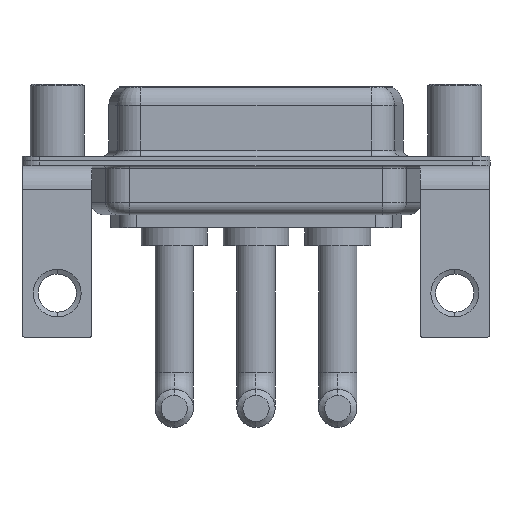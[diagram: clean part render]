
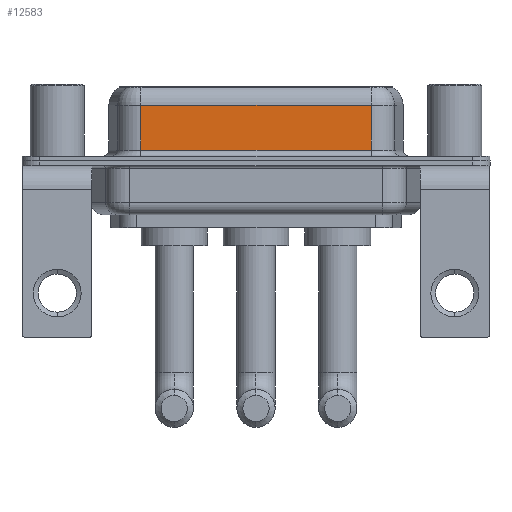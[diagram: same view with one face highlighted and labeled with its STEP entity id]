
A CAD part, front view. The second image highlights one B-rep face of the part: STEP entity #12583.
In plain terms, the highlighted planar face has unit normal (0, -1, 0).
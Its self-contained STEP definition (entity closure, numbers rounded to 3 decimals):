
#270 = VERTEX_POINT ( 'NONE', #8529 ) ;
#632 = EDGE_LOOP ( 'NONE', ( #10201, #5045, #6420, #14072 ) ) ;
#1695 = EDGE_CURVE ( 'NONE', #270, #7792, #4351, .T. ) ;
#2685 = DIRECTION ( 'NONE',  ( 0., 0., 1. ) ) ;
#2960 = CARTESIAN_POINT ( 'NONE',  ( 7.013, -3.95, 4.65 ) ) ;
#3177 = LINE ( 'NONE', #5788, #10766 ) ;
#4142 = CARTESIAN_POINT ( 'NONE',  ( 26.287, -3.95, 0.9 ) ) ;
#4351 = LINE ( 'NONE', #6605, #9673 ) ;
#4959 = AXIS2_PLACEMENT_3D ( 'NONE', #8014, #6900, #2685 ) ;
#5045 = ORIENTED_EDGE ( 'NONE', *, *, #1695, .T. ) ;
#5705 = FACE_OUTER_BOUND ( 'NONE', #632, .T. ) ;
#5788 = CARTESIAN_POINT ( 'NONE',  ( 26.287, -3.95, 6.4 ) ) ;
#6192 = EDGE_CURVE ( 'NONE', #270, #11285, #3177, .T. ) ;
#6420 = ORIENTED_EDGE ( 'NONE', *, *, #8522, .T. ) ;
#6605 = CARTESIAN_POINT ( 'NONE',  ( 26.287, -3.95, 4.65 ) ) ;
#6739 = VERTEX_POINT ( 'NONE', #7516 ) ;
#6900 = DIRECTION ( 'NONE',  ( 0., 1., 0. ) ) ;
#7064 = LINE ( 'NONE', #13915, #8185 ) ;
#7372 = LINE ( 'NONE', #9626, #10809 ) ;
#7516 = CARTESIAN_POINT ( 'NONE',  ( 7.013, -3.95, 0.9 ) ) ;
#7792 = VERTEX_POINT ( 'NONE', #2960 ) ;
#8014 = CARTESIAN_POINT ( 'NONE',  ( 26.287, -3.95, 6.4 ) ) ;
#8185 = VECTOR ( 'NONE', #14060, 1000. ) ;
#8209 = EDGE_CURVE ( 'NONE', #6739, #11285, #7372, .T. ) ;
#8522 = EDGE_CURVE ( 'NONE', #7792, #6739, #7064, .T. ) ;
#8529 = CARTESIAN_POINT ( 'NONE',  ( 26.287, -3.95, 4.65 ) ) ;
#9626 = CARTESIAN_POINT ( 'NONE',  ( 26.287, -3.95, 0.9 ) ) ;
#9673 = VECTOR ( 'NONE', #11190, 1000. ) ;
#10201 = ORIENTED_EDGE ( 'NONE', *, *, #6192, .F. ) ;
#10287 = PLANE ( 'NONE',  #4959 ) ;
#10766 = VECTOR ( 'NONE', #13325, 1000. ) ;
#10809 = VECTOR ( 'NONE', #11896, 1000. ) ;
#11190 = DIRECTION ( 'NONE',  ( -1., 0., 0. ) ) ;
#11285 = VERTEX_POINT ( 'NONE', #4142 ) ;
#11896 = DIRECTION ( 'NONE',  ( 1., 0., 0. ) ) ;
#12583 = ADVANCED_FACE ( 'NONE', ( #5705 ), #10287, .F. ) ;
#13325 = DIRECTION ( 'NONE',  ( 0., 0., -1. ) ) ;
#13915 = CARTESIAN_POINT ( 'NONE',  ( 7.013, -3.95, 6.4 ) ) ;
#14060 = DIRECTION ( 'NONE',  ( 0., 0., -1. ) ) ;
#14072 = ORIENTED_EDGE ( 'NONE', *, *, #8209, .T. ) ;
